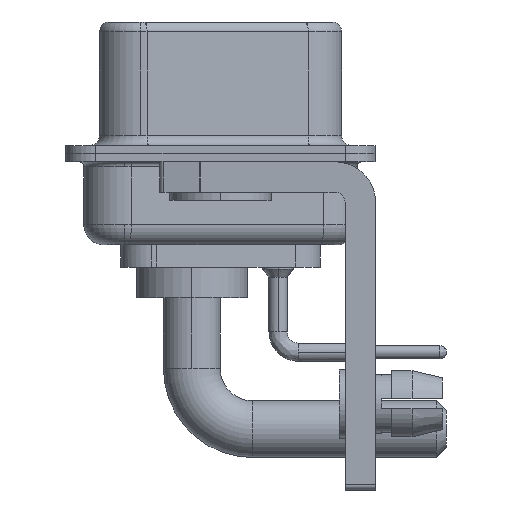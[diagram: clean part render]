
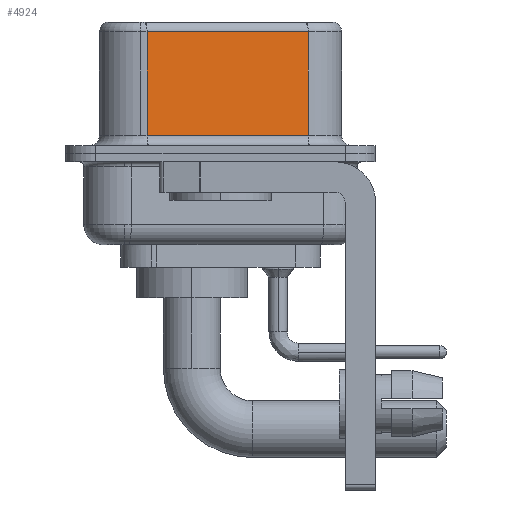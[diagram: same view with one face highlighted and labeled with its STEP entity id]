
A CAD part, left-side view. The second image highlights one B-rep face of the part: STEP entity #4924.
In plain terms, the highlighted planar face has unit normal (-0.985, -0.174, 0).
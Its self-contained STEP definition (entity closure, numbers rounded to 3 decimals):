
#395 = EDGE_CURVE ( 'NONE', #25002, #1475, #25680, .T. ) ;
#1475 = VERTEX_POINT ( 'NONE', #21293 ) ;
#2008 = EDGE_CURVE ( 'NONE', #1475, #13716, #16999, .T. ) ;
#2038 = DIRECTION ( 'NONE',  ( -0.174, 0.985, 0. ) ) ;
#3119 = ORIENTED_EDGE ( 'NONE', *, *, #2008, .T. ) ;
#3905 = AXIS2_PLACEMENT_3D ( 'NONE', #21710, #19705, #2038 ) ;
#3909 = PLANE ( 'NONE',  #3905 ) ;
#4816 = EDGE_CURVE ( 'NONE', #13716, #13334, #21447, .T. ) ;
#4875 = ORIENTED_EDGE ( 'NONE', *, *, #395, .T. ) ;
#4924 = ADVANCED_FACE ( 'NONE', ( #8143 ), #3909, .F. ) ;
#6220 = CARTESIAN_POINT ( 'NONE',  ( 3.73, 3.628, 0.9 ) ) ;
#6431 = CARTESIAN_POINT ( 'NONE',  ( 5.132, -4.322, 6.52 ) ) ;
#8143 = FACE_OUTER_BOUND ( 'NONE', #18109, .T. ) ;
#9497 = ORIENTED_EDGE ( 'NONE', *, *, #4816, .T. ) ;
#12198 = CARTESIAN_POINT ( 'NONE',  ( 5.132, -4.322, 6.02 ) ) ;
#12862 = VECTOR ( 'NONE', #15926, 1000. ) ;
#12906 = LINE ( 'NONE', #6431, #21390 ) ;
#13334 = VERTEX_POINT ( 'NONE', #22561 ) ;
#13716 = VERTEX_POINT ( 'NONE', #6220 ) ;
#14382 = DIRECTION ( 'NONE',  ( 0., 0., -1. ) ) ;
#15926 = DIRECTION ( 'NONE',  ( -0.174, 0.985, 0. ) ) ;
#16835 = ORIENTED_EDGE ( 'NONE', *, *, #20206, .F. ) ;
#16999 = LINE ( 'NONE', #25129, #18192 ) ;
#17059 = DIRECTION ( 'NONE',  ( 0.174, -0.985, 0. ) ) ;
#17256 = DIRECTION ( 'NONE',  ( 0., 0., -1. ) ) ;
#17425 = CARTESIAN_POINT ( 'NONE',  ( 5.132, -4.322, 6.02 ) ) ;
#18109 = EDGE_LOOP ( 'NONE', ( #16835, #4875, #3119, #9497 ) ) ;
#18192 = VECTOR ( 'NONE', #17256, 1000. ) ;
#19158 = VECTOR ( 'NONE', #17059, 1000. ) ;
#19705 = DIRECTION ( 'NONE',  ( 0.985, 0.174, 0. ) ) ;
#20206 = EDGE_CURVE ( 'NONE', #25002, #13334, #12906, .T. ) ;
#21293 = CARTESIAN_POINT ( 'NONE',  ( 3.73, 3.628, 6.02 ) ) ;
#21390 = VECTOR ( 'NONE', #14382, 1000. ) ;
#21447 = LINE ( 'NONE', #21576, #19158 ) ;
#21576 = CARTESIAN_POINT ( 'NONE',  ( 5.132, -4.322, 0.9 ) ) ;
#21710 = CARTESIAN_POINT ( 'NONE',  ( 5.132, -4.322, 6.52 ) ) ;
#22561 = CARTESIAN_POINT ( 'NONE',  ( 5.132, -4.322, 0.9 ) ) ;
#25002 = VERTEX_POINT ( 'NONE', #12198 ) ;
#25129 = CARTESIAN_POINT ( 'NONE',  ( 3.73, 3.628, 6.52 ) ) ;
#25680 = LINE ( 'NONE', #17425, #12862 ) ;
